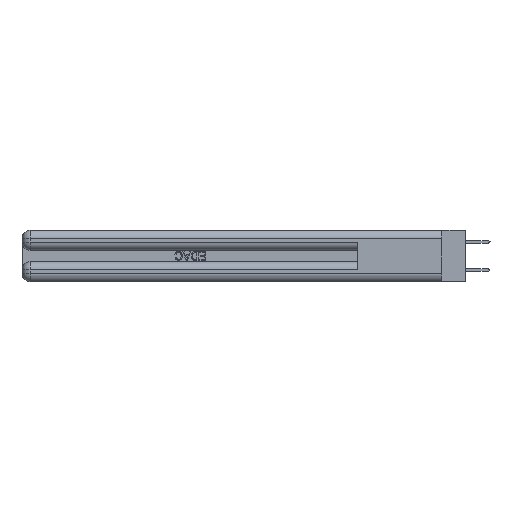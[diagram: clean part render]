
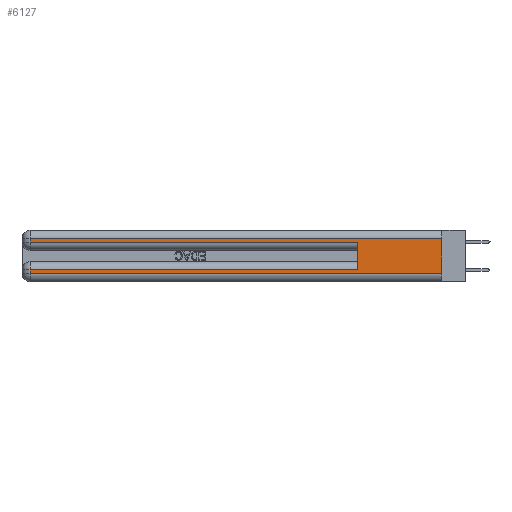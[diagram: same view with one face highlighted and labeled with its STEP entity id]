
A CAD part, left-side view. The second image highlights one B-rep face of the part: STEP entity #6127.
In plain terms, the highlighted planar face has unit normal (-1, 0, 0).
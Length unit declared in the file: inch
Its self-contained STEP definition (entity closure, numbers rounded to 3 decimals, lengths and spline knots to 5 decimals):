
#726 = DIRECTION ( 'NONE',  ( 0., 1., 0. ) ) ;
#3091 = CARTESIAN_POINT ( 'NONE',  ( 0., 2.94, 0.37 ) ) ;
#3468 = VERTEX_POINT ( 'NONE', #45063 ) ;
#4119 = EDGE_CURVE ( 'NONE', #3468, #19062, #34687, .T. ) ;
#4439 = VECTOR ( 'NONE', #25403, 39.37008 ) ;
#5382 = CARTESIAN_POINT ( 'NONE',  ( 0., 0.6, 0.145 ) ) ;
#5553 = CARTESIAN_POINT ( 'NONE',  ( 0., 2.94, 0.37 ) ) ;
#5648 = DIRECTION ( 'NONE',  ( 0., -1., 0. ) ) ;
#6127 = ADVANCED_FACE ( 'NONE', ( #18669 ), #41594, .F. ) ;
#6233 = LINE ( 'NONE', #5553, #24879 ) ;
#6437 = ORIENTED_EDGE ( 'NONE', *, *, #19358, .T. ) ;
#6513 = VERTEX_POINT ( 'NONE', #32792 ) ;
#7115 = LINE ( 'NONE', #46796, #45565 ) ;
#9899 = ORIENTED_EDGE ( 'NONE', *, *, #11164, .F. ) ;
#10115 = DIRECTION ( 'NONE',  ( 0., 0., -1. ) ) ;
#10659 = EDGE_CURVE ( 'NONE', #3468, #16539, #25796, .T. ) ;
#10720 = VERTEX_POINT ( 'NONE', #25286 ) ;
#11098 = EDGE_CURVE ( 'NONE', #10720, #16539, #38037, .T. ) ;
#11164 = EDGE_CURVE ( 'NONE', #45084, #26748, #13524, .T. ) ;
#12556 = CARTESIAN_POINT ( 'NONE',  ( 0., 0., 0.06 ) ) ;
#13524 = LINE ( 'NONE', #5382, #23411 ) ;
#15155 = ORIENTED_EDGE ( 'NONE', *, *, #4119, .T. ) ;
#15986 = VECTOR ( 'NONE', #726, 39.37008 ) ;
#16280 = DIRECTION ( 'NONE',  ( 0., -1., 0. ) ) ;
#16539 = VERTEX_POINT ( 'NONE', #40840 ) ;
#17047 = VECTOR ( 'NONE', #10115, 39.37008 ) ;
#17297 = EDGE_LOOP ( 'NONE', ( #23911, #15155, #6437, #17481, #9899, #20967, #43150, #28013 ) ) ;
#17481 = ORIENTED_EDGE ( 'NONE', *, *, #34348, .T. ) ;
#18669 = FACE_OUTER_BOUND ( 'NONE', #17297, .T. ) ;
#19062 = VERTEX_POINT ( 'NONE', #26075 ) ;
#19226 = DIRECTION ( 'NONE',  ( 1., 0., 0. ) ) ;
#19358 = EDGE_CURVE ( 'NONE', #19062, #29733, #6233, .T. ) ;
#19965 = CARTESIAN_POINT ( 'NONE',  ( 0., 2.94, 0.285 ) ) ;
#20944 = AXIS2_PLACEMENT_3D ( 'NONE', #37876, #19226, #45297 ) ;
#20967 = ORIENTED_EDGE ( 'NONE', *, *, #44550, .T. ) ;
#22669 = EDGE_CURVE ( 'NONE', #6513, #10720, #24264, .T. ) ;
#23411 = VECTOR ( 'NONE', #27692, 39.37008 ) ;
#23911 = ORIENTED_EDGE ( 'NONE', *, *, #10659, .F. ) ;
#24264 = LINE ( 'NONE', #3091, #4439 ) ;
#24879 = VECTOR ( 'NONE', #27847, 39.37008 ) ;
#25286 = CARTESIAN_POINT ( 'NONE',  ( 0., 2.94, 0.06 ) ) ;
#25403 = DIRECTION ( 'NONE',  ( 0., 0., -1. ) ) ;
#25755 = VECTOR ( 'NONE', #16280, 39.37008 ) ;
#25796 = LINE ( 'NONE', #32507, #17047 ) ;
#26075 = CARTESIAN_POINT ( 'NONE',  ( 0., 2.94, 0.31 ) ) ;
#26748 = VERTEX_POINT ( 'NONE', #38316 ) ;
#27692 = DIRECTION ( 'NONE',  ( 0., 0., 1. ) ) ;
#27847 = DIRECTION ( 'NONE',  ( 0., 0., -1. ) ) ;
#28013 = ORIENTED_EDGE ( 'NONE', *, *, #11098, .T. ) ;
#29733 = VERTEX_POINT ( 'NONE', #19965 ) ;
#32507 = CARTESIAN_POINT ( 'NONE',  ( 0., 0., 0.37 ) ) ;
#32792 = CARTESIAN_POINT ( 'NONE',  ( 0., 2.94, 0.085 ) ) ;
#34348 = EDGE_CURVE ( 'NONE', #29733, #26748, #7115, .T. ) ;
#34687 = LINE ( 'NONE', #45310, #15986 ) ;
#37876 = CARTESIAN_POINT ( 'NONE',  ( 0., 0., 0.37 ) ) ;
#38037 = LINE ( 'NONE', #12556, #25755 ) ;
#38316 = CARTESIAN_POINT ( 'NONE',  ( 0., 0.6, 0.285 ) ) ;
#40134 = CARTESIAN_POINT ( 'NONE',  ( 0., 0., 0.085 ) ) ;
#40840 = CARTESIAN_POINT ( 'NONE',  ( 0., 0., 0.06 ) ) ;
#41594 = PLANE ( 'NONE',  #20944 ) ;
#43150 = ORIENTED_EDGE ( 'NONE', *, *, #22669, .T. ) ;
#43825 = DIRECTION ( 'NONE',  ( 0., 1., 0. ) ) ;
#44278 = LINE ( 'NONE', #40134, #45459 ) ;
#44550 = EDGE_CURVE ( 'NONE', #45084, #6513, #44278, .T. ) ;
#45063 = CARTESIAN_POINT ( 'NONE',  ( 0., 0., 0.31 ) ) ;
#45084 = VERTEX_POINT ( 'NONE', #46377 ) ;
#45297 = DIRECTION ( 'NONE',  ( 0., 0., -1. ) ) ;
#45310 = CARTESIAN_POINT ( 'NONE',  ( 0., 0., 0.31 ) ) ;
#45459 = VECTOR ( 'NONE', #43825, 39.37008 ) ;
#45565 = VECTOR ( 'NONE', #5648, 39.37008 ) ;
#46377 = CARTESIAN_POINT ( 'NONE',  ( 0., 0.6, 0.085 ) ) ;
#46796 = CARTESIAN_POINT ( 'NONE',  ( 0., 0., 0.285 ) ) ;
